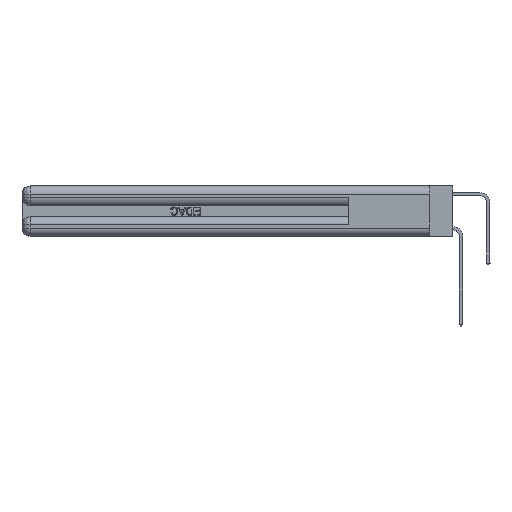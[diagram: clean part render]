
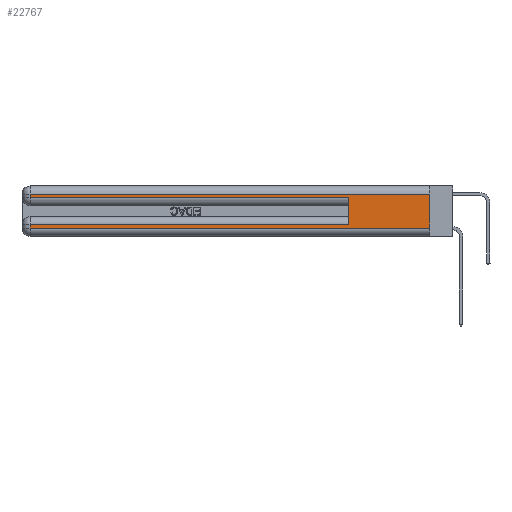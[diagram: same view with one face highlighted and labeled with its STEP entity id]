
A CAD part, left-side view. The second image highlights one B-rep face of the part: STEP entity #22767.
In plain terms, the highlighted planar face has unit normal (-1, 0, 0).
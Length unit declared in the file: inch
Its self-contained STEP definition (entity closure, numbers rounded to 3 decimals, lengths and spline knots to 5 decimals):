
#15 = CARTESIAN_POINT ( 'NONE',  ( 0., 0.6, 0.145 ) ) ;
#161 = VERTEX_POINT ( 'NONE', #464 ) ;
#428 = CARTESIAN_POINT ( 'NONE',  ( 0., 2.94, 0.285 ) ) ;
#464 = CARTESIAN_POINT ( 'NONE',  ( 0., 2.94, 0.31 ) ) ;
#634 = DIRECTION ( 'NONE',  ( 0., -1., 0. ) ) ;
#795 = EDGE_CURVE ( 'NONE', #22255, #11409, #14426, .T. ) ;
#960 = VERTEX_POINT ( 'NONE', #8576 ) ;
#1882 = VERTEX_POINT ( 'NONE', #428 ) ;
#2413 = VECTOR ( 'NONE', #15067, 39.37008 ) ;
#2628 = CARTESIAN_POINT ( 'NONE',  ( 0., 0., 0.31 ) ) ;
#3234 = VERTEX_POINT ( 'NONE', #24787 ) ;
#3607 = VERTEX_POINT ( 'NONE', #6483 ) ;
#3830 = DIRECTION ( 'NONE',  ( 1., 0., 0. ) ) ;
#6399 = ORIENTED_EDGE ( 'NONE', *, *, #10465, .F. ) ;
#6434 = FACE_OUTER_BOUND ( 'NONE', #7226, .T. ) ;
#6483 = CARTESIAN_POINT ( 'NONE',  ( 0., 0.6, 0.285 ) ) ;
#7226 = EDGE_LOOP ( 'NONE', ( #6399, #22756, #29916, #9437, #31754, #14420, #11492, #15507 ) ) ;
#7368 = EDGE_CURVE ( 'NONE', #161, #1882, #8147, .T. ) ;
#7654 = DIRECTION ( 'NONE',  ( 0., -1., 0. ) ) ;
#7983 = CARTESIAN_POINT ( 'NONE',  ( 0., 2.94, 0.37 ) ) ;
#8147 = LINE ( 'NONE', #7983, #2413 ) ;
#8209 = VECTOR ( 'NONE', #26496, 39.37008 ) ;
#8446 = DIRECTION ( 'NONE',  ( 0., 0., -1. ) ) ;
#8576 = CARTESIAN_POINT ( 'NONE',  ( 0., 0., 0.31 ) ) ;
#9202 = CARTESIAN_POINT ( 'NONE',  ( 0., 2.94, 0.06 ) ) ;
#9437 = ORIENTED_EDGE ( 'NONE', *, *, #17133, .T. ) ;
#9720 = VECTOR ( 'NONE', #19562, 39.37008 ) ;
#9946 = VECTOR ( 'NONE', #17582, 39.37008 ) ;
#10065 = CARTESIAN_POINT ( 'NONE',  ( 0., 0.6, 0.085 ) ) ;
#10465 = EDGE_CURVE ( 'NONE', #960, #3234, #27632, .T. ) ;
#10675 = EDGE_CURVE ( 'NONE', #22255, #3607, #14377, .T. ) ;
#11224 = CARTESIAN_POINT ( 'NONE',  ( 0., 2.94, 0.085 ) ) ;
#11409 = VERTEX_POINT ( 'NONE', #11224 ) ;
#11492 = ORIENTED_EDGE ( 'NONE', *, *, #16895, .T. ) ;
#12369 = VECTOR ( 'NONE', #7654, 39.37008 ) ;
#13344 = VECTOR ( 'NONE', #634, 39.37008 ) ;
#13676 = CARTESIAN_POINT ( 'NONE',  ( 0., 0., 0.37 ) ) ;
#13944 = LINE ( 'NONE', #28480, #26803 ) ;
#14284 = VERTEX_POINT ( 'NONE', #9202 ) ;
#14377 = LINE ( 'NONE', #15, #8209 ) ;
#14420 = ORIENTED_EDGE ( 'NONE', *, *, #795, .T. ) ;
#14426 = LINE ( 'NONE', #14582, #9946 ) ;
#14582 = CARTESIAN_POINT ( 'NONE',  ( 0., 0., 0.085 ) ) ;
#14748 = AXIS2_PLACEMENT_3D ( 'NONE', #13676, #3830, #22894 ) ;
#14866 = LINE ( 'NONE', #2628, #9720 ) ;
#15067 = DIRECTION ( 'NONE',  ( 0., 0., -1. ) ) ;
#15507 = ORIENTED_EDGE ( 'NONE', *, *, #25619, .T. ) ;
#15672 = CARTESIAN_POINT ( 'NONE',  ( 0., 0., 0.37 ) ) ;
#16895 = EDGE_CURVE ( 'NONE', #11409, #14284, #13944, .T. ) ;
#17133 = EDGE_CURVE ( 'NONE', #1882, #3607, #27797, .T. ) ;
#17582 = DIRECTION ( 'NONE',  ( 0., 1., 0. ) ) ;
#19562 = DIRECTION ( 'NONE',  ( 0., 1., 0. ) ) ;
#20527 = VECTOR ( 'NONE', #8446, 39.37008 ) ;
#22255 = VERTEX_POINT ( 'NONE', #10065 ) ;
#22747 = CARTESIAN_POINT ( 'NONE',  ( 0., 0., 0.06 ) ) ;
#22756 = ORIENTED_EDGE ( 'NONE', *, *, #24898, .T. ) ;
#22767 = ADVANCED_FACE ( 'NONE', ( #6434 ), #30927, .F. ) ;
#22894 = DIRECTION ( 'NONE',  ( 0., 0., -1. ) ) ;
#23062 = LINE ( 'NONE', #22747, #13344 ) ;
#24787 = CARTESIAN_POINT ( 'NONE',  ( 0., 0., 0.06 ) ) ;
#24898 = EDGE_CURVE ( 'NONE', #960, #161, #14866, .T. ) ;
#25386 = CARTESIAN_POINT ( 'NONE',  ( 0., 0., 0.285 ) ) ;
#25619 = EDGE_CURVE ( 'NONE', #14284, #3234, #23062, .T. ) ;
#26496 = DIRECTION ( 'NONE',  ( 0., 0., 1. ) ) ;
#26803 = VECTOR ( 'NONE', #28159, 39.37008 ) ;
#27632 = LINE ( 'NONE', #15672, #20527 ) ;
#27797 = LINE ( 'NONE', #25386, #12369 ) ;
#28159 = DIRECTION ( 'NONE',  ( 0., 0., -1. ) ) ;
#28480 = CARTESIAN_POINT ( 'NONE',  ( 0., 2.94, 0.37 ) ) ;
#29916 = ORIENTED_EDGE ( 'NONE', *, *, #7368, .T. ) ;
#30927 = PLANE ( 'NONE',  #14748 ) ;
#31754 = ORIENTED_EDGE ( 'NONE', *, *, #10675, .F. ) ;
